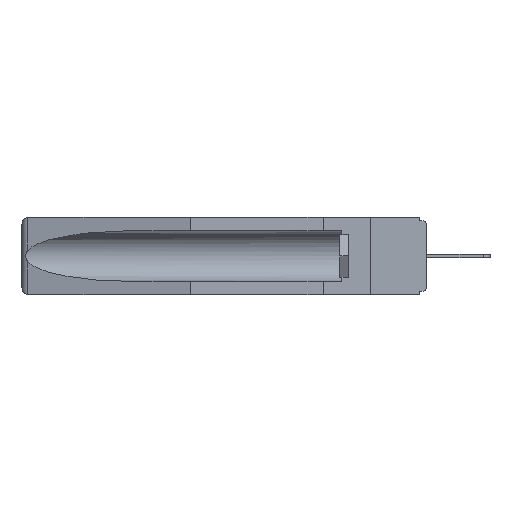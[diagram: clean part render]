
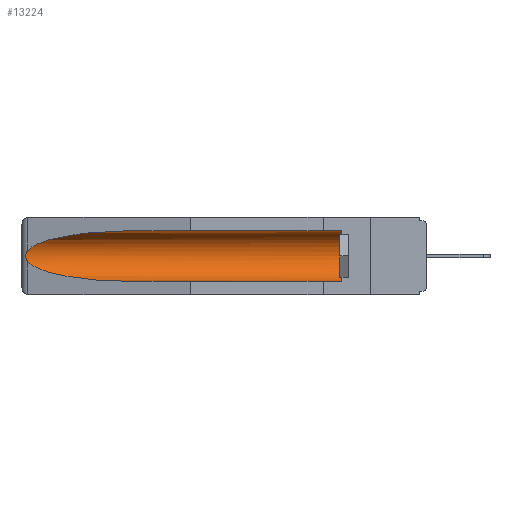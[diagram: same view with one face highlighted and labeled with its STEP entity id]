
A CAD part, left-side view. The second image highlights one B-rep face of the part: STEP entity #13224.
In plain terms, the highlighted cylindrical face has radius 2.857 mm (diameter 5.715 mm), a partial arc.
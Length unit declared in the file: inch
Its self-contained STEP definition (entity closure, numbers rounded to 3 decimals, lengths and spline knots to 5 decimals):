
#89 = LINE ( 'NONE', #5811, #1762 ) ;
#227 = EDGE_CURVE ( 'NONE', #6445, #15758, #11104, .T. ) ;
#647 = DIRECTION ( 'NONE',  ( 0., -1., 0. ) ) ;
#1048 = CARTESIAN_POINT ( 'NONE',  ( 0.2675, 1.53308, -0.17534 ) ) ;
#1354 = CARTESIAN_POINT ( 'NONE',  ( 0.25451, 1.48313, -0.24835 ) ) ;
#1428 = CARTESIAN_POINT ( 'NONE',  ( 0.26537, 1.52718, -0.19328 ) ) ;
#1495 = ORIENTED_EDGE ( 'NONE', *, *, #227, .T. ) ;
#1619 = ORIENTED_EDGE ( 'NONE', *, *, #14178, .T. ) ;
#1762 = VECTOR ( 'NONE', #4313, 39.37008 ) ;
#1804 = ORIENTED_EDGE ( 'NONE', *, *, #14346, .T. ) ;
#1814 = VERTEX_POINT ( 'NONE', #7761 ) ;
#2071 = EDGE_CURVE ( 'NONE', #6432, #15758, #89, .T. ) ;
#2298 = CARTESIAN_POINT ( 'NONE',  ( 0.26597, 1.5296, -0.19026 ) ) ;
#2615 = CARTESIAN_POINT ( 'NONE',  ( 0.26537, 1.52718, -0.19328 ) ) ;
#3164 = ORIENTED_EDGE ( 'NONE', *, *, #2071, .F. ) ;
#4117 = CARTESIAN_POINT ( 'NONE',  ( 0.155, 1.07973, -0.284 ) ) ;
#4313 = DIRECTION ( 'NONE',  ( 0., 1., 0. ) ) ;
#4814 = VECTOR ( 'NONE', #16067, 39.37008 ) ;
#5381 = CARTESIAN_POINT ( 'NONE',  ( 0.155, 0.126, -0.059 ) ) ;
#5598 = CARTESIAN_POINT ( 'NONE',  ( 0.25451, 1.48313, -0.09465 ) ) ;
#5811 = CARTESIAN_POINT ( 'NONE',  ( 0.155, -0.30754, -0.284 ) ) ;
#5989 = CARTESIAN_POINT ( 'NONE',  ( 0.155, 1.07973, -0.284 ) ) ;
#6222 = DIRECTION ( 'NONE',  ( 0., 1., 0. ) ) ;
#6273 = CARTESIAN_POINT ( 'NONE',  ( 0.26597, 1.52961, -0.15275 ) ) ;
#6432 = VERTEX_POINT ( 'NONE', #9651 ) ;
#6445 = VERTEX_POINT ( 'NONE', #1428 ) ;
#6564 = AXIS2_PLACEMENT_3D ( 'NONE', #11554, #647, #12752 ) ;
#6841 = CARTESIAN_POINT ( 'NONE',  ( 0.155, 1.07973, -0.059 ) ) ;
#6924 =( BOUNDED_CURVE ( )  B_SPLINE_CURVE ( 3, ( #6841, #13838, #5598, #16378 ),
 .UNSPECIFIED., .F., .F. ) 
 B_SPLINE_CURVE_WITH_KNOTS ( ( 4, 4 ),
 ( 4.71239, 6.08839 ),
 .UNSPECIFIED. ) 
 CURVE ( )  GEOMETRIC_REPRESENTATION_ITEM ( )  RATIONAL_B_SPLINE_CURVE ( ( 1., 0.848, 0.848, 1. ) ) 
 REPRESENTATION_ITEM ( '' )  );
#7565 = ORIENTED_EDGE ( 'NONE', *, *, #16040, .T. ) ;
#7633 = CIRCLE ( 'NONE', #6564, 0.1125 ) ;
#7761 = CARTESIAN_POINT ( 'NONE',  ( 0.155, 1.07973, -0.059 ) ) ;
#7979 = CARTESIAN_POINT ( 'NONE',  ( 0.2673, 1.53269, -0.17917 ) ) ;
#8213 = B_SPLINE_CURVE_WITH_KNOTS ( 'NONE', 3,
 ( #14443, #6273, #15827, #15878, #12103, #1048, #7979, #14697, #2298, #11921 ),
 .UNSPECIFIED., .F., .F.,
 ( 4, 2, 2, 2, 4 ),
 ( 0., 0.00029, 0.00058, 0.00087, 0.00117 ),
 .UNSPECIFIED. ) ;
#8422 = LINE ( 'NONE', #9403, #4814 ) ;
#9021 = CARTESIAN_POINT ( 'NONE',  ( 0.155, -0.30754, -0.1715 ) ) ;
#9403 = CARTESIAN_POINT ( 'NONE',  ( 0.155, -0.30754, -0.059 ) ) ;
#9478 = VERTEX_POINT ( 'NONE', #5381 ) ;
#9651 = CARTESIAN_POINT ( 'NONE',  ( 0.155, 0.126, -0.284 ) ) ;
#10721 = CARTESIAN_POINT ( 'NONE',  ( 0.26537, 1.52718, -0.14972 ) ) ;
#11104 =( BOUNDED_CURVE ( )  B_SPLINE_CURVE ( 3, ( #2615, #1354, #17682, #4117 ),
 .UNSPECIFIED., .F., .F. ) 
 B_SPLINE_CURVE_WITH_KNOTS ( ( 4, 4 ),
 ( 0.1948, 1.5708 ),
 .UNSPECIFIED. ) 
 CURVE ( )  GEOMETRIC_REPRESENTATION_ITEM ( )  RATIONAL_B_SPLINE_CURVE ( ( 1., 0.848, 0.848, 1. ) ) 
 REPRESENTATION_ITEM ( '' )  );
#11487 = AXIS2_PLACEMENT_3D ( 'NONE', #9021, #6222, #15775 ) ;
#11554 = CARTESIAN_POINT ( 'NONE',  ( 0.155, 0.126, -0.1715 ) ) ;
#11607 = EDGE_CURVE ( 'NONE', #9478, #1814, #8422, .T. ) ;
#11921 = CARTESIAN_POINT ( 'NONE',  ( 0.26537, 1.52718, -0.19328 ) ) ;
#11945 = ORIENTED_EDGE ( 'NONE', *, *, #11607, .T. ) ;
#12103 = CARTESIAN_POINT ( 'NONE',  ( 0.2675, 1.53308, -0.16763 ) ) ;
#12692 = CYLINDRICAL_SURFACE ( 'NONE', #11487, 0.1125 ) ;
#12752 = DIRECTION ( 'NONE',  ( 0., 0., 1. ) ) ;
#13101 = FACE_OUTER_BOUND ( 'NONE', #13416, .T. ) ;
#13224 = ADVANCED_FACE ( 'NONE', ( #13101 ), #12692, .F. ) ;
#13416 = EDGE_LOOP ( 'NONE', ( #1804, #1619, #1495, #3164, #7565, #11945 ) ) ;
#13838 = CARTESIAN_POINT ( 'NONE',  ( 0.21114, 1.30732, -0.059 ) ) ;
#14178 = EDGE_CURVE ( 'NONE', #17062, #6445, #8213, .T. ) ;
#14346 = EDGE_CURVE ( 'NONE', #1814, #17062, #6924, .T. ) ;
#14443 = CARTESIAN_POINT ( 'NONE',  ( 0.26537, 1.52718, -0.14972 ) ) ;
#14697 = CARTESIAN_POINT ( 'NONE',  ( 0.26655, 1.53094, -0.18657 ) ) ;
#15758 = VERTEX_POINT ( 'NONE', #5989 ) ;
#15775 = DIRECTION ( 'NONE',  ( 0., 0., 1. ) ) ;
#15827 = CARTESIAN_POINT ( 'NONE',  ( 0.26654, 1.53092, -0.15636 ) ) ;
#15878 = CARTESIAN_POINT ( 'NONE',  ( 0.2673, 1.5327, -0.16383 ) ) ;
#16040 = EDGE_CURVE ( 'NONE', #6432, #9478, #7633, .T. ) ;
#16067 = DIRECTION ( 'NONE',  ( 0., 1., 0. ) ) ;
#16378 = CARTESIAN_POINT ( 'NONE',  ( 0.26537, 1.52718, -0.14972 ) ) ;
#17062 = VERTEX_POINT ( 'NONE', #10721 ) ;
#17682 = CARTESIAN_POINT ( 'NONE',  ( 0.21114, 1.30732, -0.284 ) ) ;
